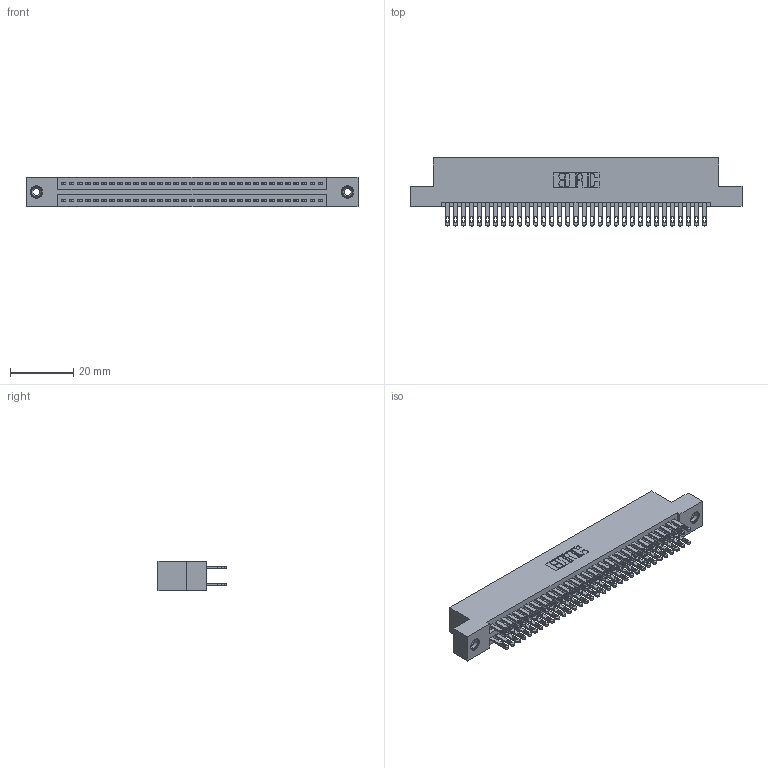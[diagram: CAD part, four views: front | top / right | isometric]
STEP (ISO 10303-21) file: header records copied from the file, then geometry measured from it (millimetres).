
FILE_DESCRIPTION (( 'STEP AP203' ), '1' );
FILE_NAME ('345-066-500-208.STEP', '2019-10-30T15:49:26', ( '' ), ( '' ), 'SwSTEP 2.0', 'SolidWorks 2016', '' );
FILE_SCHEMA (( 'CONFIG_CONTROL_DESIGN' ));
Length unit declared in the file: inch
Products named in the file (4): 345-066-500-208; 345 Part_Flush Mounting Lugs - 0.156 Dia-TI; 345-250-001_345-250-003-102; 345-292-001_345-293-100
Assembly tree (69 placements, depth 2):
  345-066-500-208
    345 Part_Flush Mounting Lugs - 0.156 Dia-TI
    345-292-001_345-293-100  x66
    345-250-001_345-250-003-102  x2
Bounding box: 105.03 x 21.51 x 9.4 mm (x, y, z)
Volume: 10314.3 mm3; surface area: 15758.5 mm2
Topology: 69 solids, 69 shells, 3222 faces, 9783 edges, 6514 vertices
Faces by surface type: plane 1894, cylinder 1312, cone 12, torus 4
Entity records: 28220 total; most frequent: CARTESIAN_POINT 4719, ORIENTED_EDGE 4646, DIRECTION 4201, EDGE_CURVE 2323, VECTOR 2035, LINE 2035, VERTEX_POINT 1544, AXIS2_PLACEMENT_3D 1083
